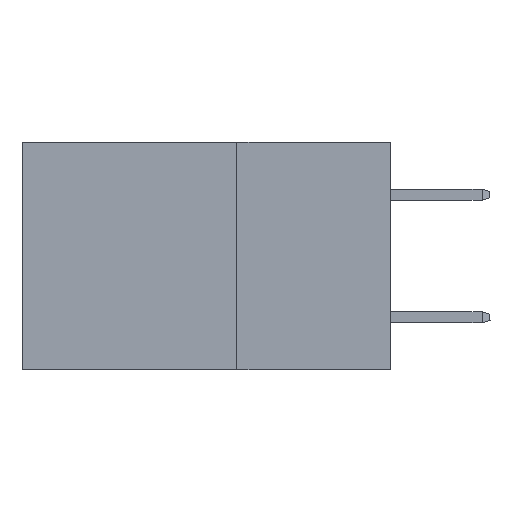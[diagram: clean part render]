
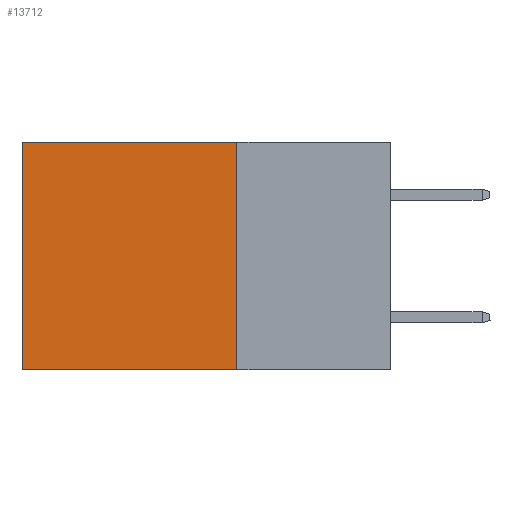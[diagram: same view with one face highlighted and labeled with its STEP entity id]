
A CAD part, left-side view. The second image highlights one B-rep face of the part: STEP entity #13712.
In plain terms, the highlighted planar face has unit normal (-1, 0, 0).
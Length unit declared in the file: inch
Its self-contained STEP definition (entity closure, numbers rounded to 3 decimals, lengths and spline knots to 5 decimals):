
#911 = EDGE_LOOP ( 'NONE', ( #12176, #8608, #16117, #21486 ) ) ;
#2062 = CARTESIAN_POINT ( 'NONE',  ( 0.2875, 0.25, 0. ) ) ;
#2180 = VERTEX_POINT ( 'NONE', #15564 ) ;
#2409 = EDGE_CURVE ( 'NONE', #20527, #22761, #23568, .T. ) ;
#2494 = CARTESIAN_POINT ( 'NONE',  ( 0.2875, 0.25, 0. ) ) ;
#3227 = CARTESIAN_POINT ( 'NONE',  ( 0.2875, 0.6, 0. ) ) ;
#3859 = DIRECTION ( 'NONE',  ( 0., 0., -1. ) ) ;
#4589 = LINE ( 'NONE', #20899, #23717 ) ;
#5033 = VECTOR ( 'NONE', #3859, 39.37008 ) ;
#5057 = EDGE_CURVE ( 'NONE', #19080, #2180, #17676, .T. ) ;
#6251 = PLANE ( 'NONE',  #16796 ) ;
#7808 = VECTOR ( 'NONE', #10661, 39.37008 ) ;
#7844 = CARTESIAN_POINT ( 'NONE',  ( 0.2875, 0.25, -0.37 ) ) ;
#8020 = DIRECTION ( 'NONE',  ( 1., 0., 0. ) ) ;
#8608 = ORIENTED_EDGE ( 'NONE', *, *, #8912, .F. ) ;
#8912 = EDGE_CURVE ( 'NONE', #22761, #2180, #9265, .T. ) ;
#9265 = LINE ( 'NONE', #7844, #23769 ) ;
#9667 = CARTESIAN_POINT ( 'NONE',  ( 0.2875, 0.25, 0. ) ) ;
#9901 = DIRECTION ( 'NONE',  ( 0., 0., -1. ) ) ;
#10661 = DIRECTION ( 'NONE',  ( 0., 0., -1. ) ) ;
#11837 = DIRECTION ( 'NONE',  ( 0., 1., 0. ) ) ;
#12176 = ORIENTED_EDGE ( 'NONE', *, *, #5057, .T. ) ;
#13466 = DIRECTION ( 'NONE',  ( 0., 1., 0. ) ) ;
#13712 = ADVANCED_FACE ( 'NONE', ( #13962 ), #6251, .F. ) ;
#13962 = FACE_OUTER_BOUND ( 'NONE', #911, .T. ) ;
#15564 = CARTESIAN_POINT ( 'NONE',  ( 0.2875, 0.6, -0.37 ) ) ;
#16117 = ORIENTED_EDGE ( 'NONE', *, *, #2409, .F. ) ;
#16796 = AXIS2_PLACEMENT_3D ( 'NONE', #2494, #8020, #9901 ) ;
#17676 = LINE ( 'NONE', #3227, #7808 ) ;
#19080 = VERTEX_POINT ( 'NONE', #23477 ) ;
#19323 = EDGE_CURVE ( 'NONE', #20527, #19080, #4589, .T. ) ;
#19942 = CARTESIAN_POINT ( 'NONE',  ( 0.2875, 0.25, -0.37 ) ) ;
#20527 = VERTEX_POINT ( 'NONE', #2062 ) ;
#20899 = CARTESIAN_POINT ( 'NONE',  ( 0.2875, 0.25, 0. ) ) ;
#21486 = ORIENTED_EDGE ( 'NONE', *, *, #19323, .T. ) ;
#22761 = VERTEX_POINT ( 'NONE', #19942 ) ;
#23477 = CARTESIAN_POINT ( 'NONE',  ( 0.2875, 0.6, 0. ) ) ;
#23568 = LINE ( 'NONE', #9667, #5033 ) ;
#23717 = VECTOR ( 'NONE', #11837, 39.37008 ) ;
#23769 = VECTOR ( 'NONE', #13466, 39.37008 ) ;
